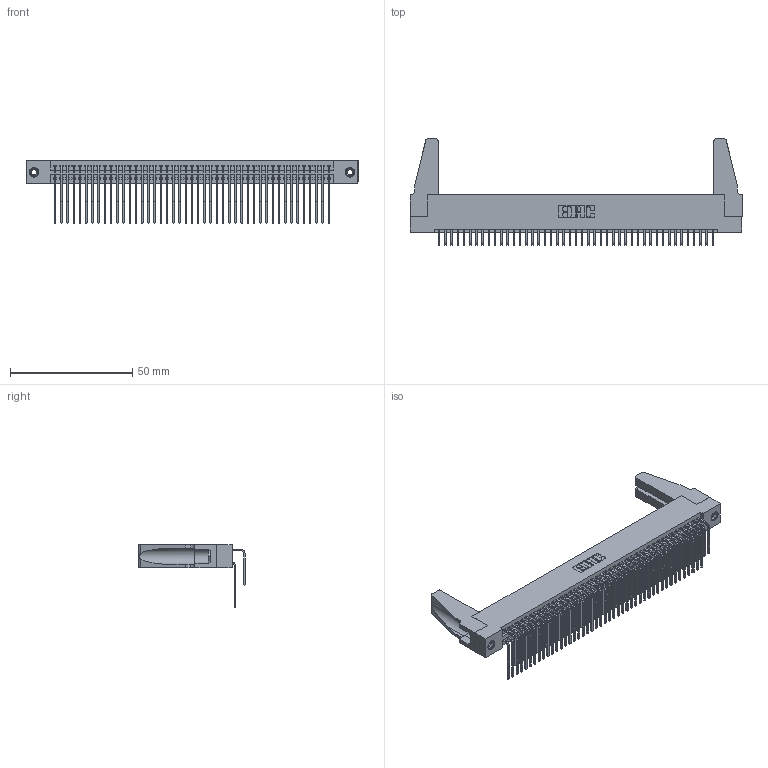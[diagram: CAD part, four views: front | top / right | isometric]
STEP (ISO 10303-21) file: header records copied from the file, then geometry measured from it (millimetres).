
FILE_DESCRIPTION (( 'STEP AP203' ), '1' );
FILE_NAME ('395-090-559-288.STEP', '2019-10-25T17:59:02', ( '' ), ( '' ), 'SwSTEP 2.0', 'SolidWorks 2016', '' );
FILE_SCHEMA (( 'CONFIG_CONTROL_DESIGN' ));
Length unit declared in the file: inch
Products named in the file (6): 345 Part_Flush Mounting Lugs - 0.156 Dia-TH; 345-292-001_558 559 Tail - 1; 345-292-001_559 Tail - 2; 345-250-001_345-250-001-102; 345-220-078_345-220-088; 395-090-559-288
Assembly tree (95 placements, depth 2):
  395-090-559-288
    345 Part_Flush Mounting Lugs - 0.156 Dia-TH
    345-292-001_558 559 Tail - 1  x45
    345-292-001_559 Tail - 2  x45
    345-250-001_345-250-001-102  x2
    345-220-078_345-220-088  x2
Bounding box: 135.53 x 43.42 x 25.53 mm (x, y, z)
Volume: 16965.4 mm3; surface area: 25891.7 mm2
Topology: 95 solids, 95 shells, 4930 faces, 14605 edges, 9606 vertices
Faces by surface type: plane 3302, cylinder 1612, cone 12, torus 4
Entity records: 38704 total; most frequent: CARTESIAN_POINT 6525, ORIENTED_EDGE 6368, DIRECTION 5728, EDGE_CURVE 3184, VECTOR 2790, LINE 2790, VERTEX_POINT 2114, AXIS2_PLACEMENT_3D 1469
